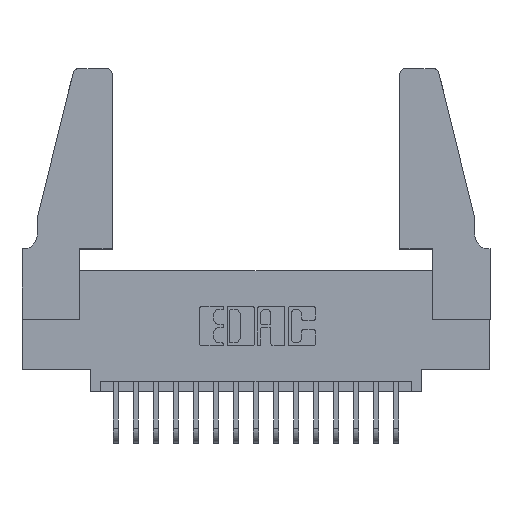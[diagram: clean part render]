
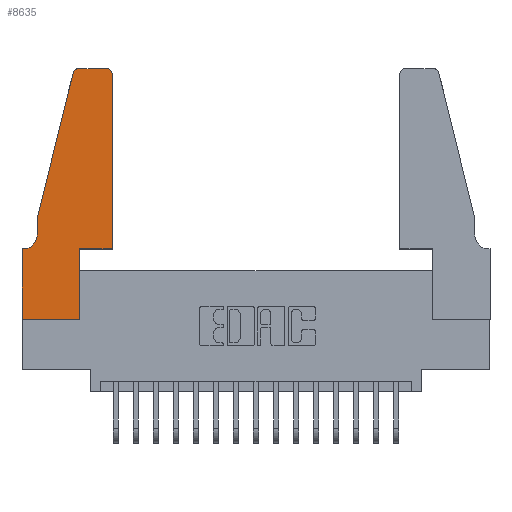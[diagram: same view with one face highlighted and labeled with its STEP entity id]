
A CAD part, top view. The second image highlights one B-rep face of the part: STEP entity #8635.
In plain terms, the highlighted planar face has unit normal (0, 0, 1).
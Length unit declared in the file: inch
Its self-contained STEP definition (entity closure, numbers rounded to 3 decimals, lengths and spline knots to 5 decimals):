
#234 = EDGE_CURVE ( 'NONE', #12284, #12234, #8305, .T. ) ;
#604 = ORIENTED_EDGE ( 'NONE', *, *, #19011, .T. ) ;
#761 = DIRECTION ( 'NONE',  ( 1., 0., 0. ) ) ;
#940 = CARTESIAN_POINT ( 'NONE',  ( 0.2605, 1.25, 0.37 ) ) ;
#1366 = CARTESIAN_POINT ( 'NONE',  ( 0.0755, 0.5, 0.37 ) ) ;
#1452 = CARTESIAN_POINT ( 'NONE',  ( 0.0755, 0.42, 0.37 ) ) ;
#1529 = DIRECTION ( 'NONE',  ( 1., 0., 0. ) ) ;
#1579 = DIRECTION ( 'NONE',  ( 0., -1., 0. ) ) ;
#1911 = VECTOR ( 'NONE', #16132, 39.37008 ) ;
#1946 = EDGE_CURVE ( 'NONE', #5532, #10905, #1969, .T. ) ;
#1969 = LINE ( 'NONE', #9794, #11359 ) ;
#2478 = VERTEX_POINT ( 'NONE', #1366 ) ;
#2658 = ORIENTED_EDGE ( 'NONE', *, *, #9971, .T. ) ;
#2734 = VECTOR ( 'NONE', #1579, 39.37008 ) ;
#2895 = CARTESIAN_POINT ( 'NONE',  ( 0.0755, 0.5, 0.37 ) ) ;
#2974 = CARTESIAN_POINT ( 'NONE',  ( 0.25487, 1.22718, 0.37 ) ) ;
#3097 = CARTESIAN_POINT ( 'NONE',  ( 0.284, 1.22, 0.37 ) ) ;
#3225 = AXIS2_PLACEMENT_3D ( 'NONE', #3686, #6558, #14155 ) ;
#3268 = CARTESIAN_POINT ( 'NONE',  ( 0.2865, 0., 0.37 ) ) ;
#3469 = AXIS2_PLACEMENT_3D ( 'NONE', #3097, #4609, #1529 ) ;
#3686 = CARTESIAN_POINT ( 'NONE',  ( 0., 0.35, 0.37 ) ) ;
#3717 = VECTOR ( 'NONE', #12449, 39.37008 ) ;
#4266 = AXIS2_PLACEMENT_3D ( 'NONE', #6381, #10809, #15343 ) ;
#4408 = LINE ( 'NONE', #4856, #3717 ) ;
#4609 = DIRECTION ( 'NONE',  ( 0., 0., 1. ) ) ;
#4826 = CARTESIAN_POINT ( 'NONE',  ( 0., 0., 0.37 ) ) ;
#4856 = CARTESIAN_POINT ( 'NONE',  ( 0.4505, 0.35, 0.37 ) ) ;
#4894 = VECTOR ( 'NONE', #6115, 39.37008 ) ;
#4921 = VECTOR ( 'NONE', #10908, 39.37008 ) ;
#5084 = VERTEX_POINT ( 'NONE', #8307 ) ;
#5110 = CIRCLE ( 'NONE', #3469, 0.03 ) ;
#5317 = EDGE_CURVE ( 'NONE', #8539, #15092, #4408, .T. ) ;
#5532 = VERTEX_POINT ( 'NONE', #17440 ) ;
#5576 = CARTESIAN_POINT ( 'NONE',  ( 0.2865, 0.35, 0.37 ) ) ;
#5733 = EDGE_CURVE ( 'NONE', #5084, #12381, #5110, .T. ) ;
#5933 = CARTESIAN_POINT ( 'NONE',  ( 0.4505, 0.35, 0.37 ) ) ;
#5956 = ORIENTED_EDGE ( 'NONE', *, *, #18429, .T. ) ;
#5965 = EDGE_CURVE ( 'NONE', #15482, #8539, #8587, .T. ) ;
#6115 = DIRECTION ( 'NONE',  ( 1., 0., 0. ) ) ;
#6381 = CARTESIAN_POINT ( 'NONE',  ( 0.0055, 0.42, 0.37 ) ) ;
#6558 = DIRECTION ( 'NONE',  ( 0., 0., 1. ) ) ;
#6625 = PLANE ( 'NONE',  #3225 ) ;
#6721 = LINE ( 'NONE', #2895, #2734 ) ;
#7019 = ORIENTED_EDGE ( 'NONE', *, *, #234, .T. ) ;
#7439 = CARTESIAN_POINT ( 'NONE',  ( 0.4505, 0.35, 0.37 ) ) ;
#7573 = DIRECTION ( 'NONE',  ( 0., 1., 0. ) ) ;
#7689 = LINE ( 'NONE', #4826, #4894 ) ;
#8190 = ORIENTED_EDGE ( 'NONE', *, *, #13296, .T. ) ;
#8305 = CIRCLE ( 'NONE', #15355, 0.03 ) ;
#8307 = CARTESIAN_POINT ( 'NONE',  ( 0.284, 1.25, 0.37 ) ) ;
#8539 = VERTEX_POINT ( 'NONE', #5576 ) ;
#8587 = LINE ( 'NONE', #9652, #10012 ) ;
#8635 = ADVANCED_FACE ( 'NONE', ( #11316 ), #6625, .T. ) ;
#8943 = EDGE_CURVE ( 'NONE', #12381, #2478, #12226, .T. ) ;
#9390 = ORIENTED_EDGE ( 'NONE', *, *, #8943, .T. ) ;
#9600 = ORIENTED_EDGE ( 'NONE', *, *, #1946, .T. ) ;
#9652 = CARTESIAN_POINT ( 'NONE',  ( 0.2865, 0.35, 0.37 ) ) ;
#9738 = CARTESIAN_POINT ( 'NONE',  ( 0.4205, 1.22, 0.37 ) ) ;
#9794 = CARTESIAN_POINT ( 'NONE',  ( 0.0755, 0.35, 0.37 ) ) ;
#9971 = EDGE_CURVE ( 'NONE', #10905, #15886, #13091, .T. ) ;
#10012 = VECTOR ( 'NONE', #11183, 39.37008 ) ;
#10091 = EDGE_CURVE ( 'NONE', #12234, #5084, #11035, .T. ) ;
#10094 = ORIENTED_EDGE ( 'NONE', *, *, #11511, .T. ) ;
#10436 = CARTESIAN_POINT ( 'NONE',  ( 0.4505, 1.22, 0.37 ) ) ;
#10779 = LINE ( 'NONE', #7439, #14696 ) ;
#10809 = DIRECTION ( 'NONE',  ( 0., 0., -1. ) ) ;
#10905 = VERTEX_POINT ( 'NONE', #15350 ) ;
#10908 = DIRECTION ( 'NONE',  ( 0., -1., 0. ) ) ;
#11035 = LINE ( 'NONE', #940, #11489 ) ;
#11183 = DIRECTION ( 'NONE',  ( 0., 1., 0. ) ) ;
#11316 = FACE_OUTER_BOUND ( 'NONE', #17726, .T. ) ;
#11359 = VECTOR ( 'NONE', #15783, 39.37008 ) ;
#11489 = VECTOR ( 'NONE', #14588, 39.37008 ) ;
#11511 = EDGE_CURVE ( 'NONE', #14021, #5532, #12005, .T. ) ;
#11823 = CARTESIAN_POINT ( 'NONE',  ( 0.0755, 0.5, 0.37 ) ) ;
#11995 = CARTESIAN_POINT ( 'NONE',  ( 0., 0., 0.37 ) ) ;
#12005 = CIRCLE ( 'NONE', #4266, 0.07 ) ;
#12226 = LINE ( 'NONE', #11823, #1911 ) ;
#12234 = VERTEX_POINT ( 'NONE', #16968 ) ;
#12284 = VERTEX_POINT ( 'NONE', #10436 ) ;
#12345 = ORIENTED_EDGE ( 'NONE', *, *, #5733, .T. ) ;
#12381 = VERTEX_POINT ( 'NONE', #2974 ) ;
#12449 = DIRECTION ( 'NONE',  ( 1., 0., 0. ) ) ;
#13054 = DIRECTION ( 'NONE',  ( 0., 0., 1. ) ) ;
#13091 = LINE ( 'NONE', #11995, #4921 ) ;
#13296 = EDGE_CURVE ( 'NONE', #15092, #12284, #10779, .T. ) ;
#14021 = VERTEX_POINT ( 'NONE', #1452 ) ;
#14155 = DIRECTION ( 'NONE',  ( 1., 0., 0. ) ) ;
#14588 = DIRECTION ( 'NONE',  ( -1., 0., 0. ) ) ;
#14676 = ORIENTED_EDGE ( 'NONE', *, *, #10091, .T. ) ;
#14696 = VECTOR ( 'NONE', #7573, 39.37008 ) ;
#15092 = VERTEX_POINT ( 'NONE', #5933 ) ;
#15343 = DIRECTION ( 'NONE',  ( -1., 0., 0. ) ) ;
#15350 = CARTESIAN_POINT ( 'NONE',  ( 0., 0.35, 0.37 ) ) ;
#15355 = AXIS2_PLACEMENT_3D ( 'NONE', #9738, #13054, #761 ) ;
#15482 = VERTEX_POINT ( 'NONE', #3268 ) ;
#15783 = DIRECTION ( 'NONE',  ( -1., 0., 0. ) ) ;
#15886 = VERTEX_POINT ( 'NONE', #16000 ) ;
#16000 = CARTESIAN_POINT ( 'NONE',  ( 0., 0., 0.37 ) ) ;
#16132 = DIRECTION ( 'NONE',  ( -0.239, -0.971, 0. ) ) ;
#16968 = CARTESIAN_POINT ( 'NONE',  ( 0.4205, 1.25, 0.37 ) ) ;
#17440 = CARTESIAN_POINT ( 'NONE',  ( 0.0055, 0.35, 0.37 ) ) ;
#17726 = EDGE_LOOP ( 'NONE', ( #14676, #12345, #9390, #604, #10094, #9600, #2658, #5956, #18046, #18675, #8190, #7019 ) ) ;
#18046 = ORIENTED_EDGE ( 'NONE', *, *, #5965, .T. ) ;
#18429 = EDGE_CURVE ( 'NONE', #15886, #15482, #7689, .T. ) ;
#18675 = ORIENTED_EDGE ( 'NONE', *, *, #5317, .T. ) ;
#19011 = EDGE_CURVE ( 'NONE', #2478, #14021, #6721, .T. ) ;
